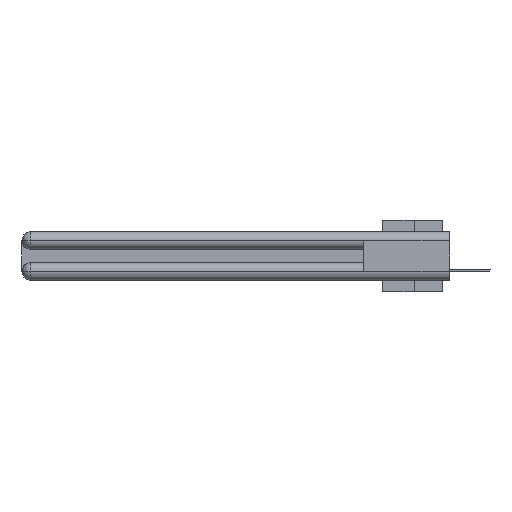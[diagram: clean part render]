
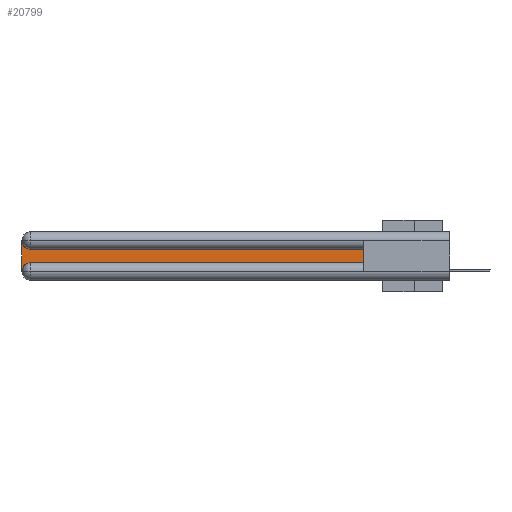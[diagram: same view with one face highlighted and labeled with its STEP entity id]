
A CAD part, left-side view. The second image highlights one B-rep face of the part: STEP entity #20799.
In plain terms, the highlighted planar face has unit normal (-1, 0, 0).
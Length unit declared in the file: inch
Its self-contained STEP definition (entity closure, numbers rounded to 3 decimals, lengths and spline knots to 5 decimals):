
#950 = VERTEX_POINT ( 'NONE', #7130 ) ;
#980 = EDGE_CURVE ( 'NONE', #950, #35146, #34189, .T. ) ;
#1785 = DIRECTION ( 'NONE',  ( 0., 0., -1. ) ) ;
#2163 = PLANE ( 'NONE',  #35764 ) ;
#2497 = CARTESIAN_POINT ( 'NONE',  ( 0.075, 2.94, -0.2175 ) ) ;
#3583 = VECTOR ( 'NONE', #12370, 39.37008 ) ;
#4427 = EDGE_CURVE ( 'NONE', #16533, #14199, #17996, .T. ) ;
#4843 = DIRECTION ( 'NONE',  ( 1., 0., 0. ) ) ;
#4846 = DIRECTION ( 'NONE',  ( 1., 0., 0. ) ) ;
#6538 = ORIENTED_EDGE ( 'NONE', *, *, #980, .T. ) ;
#7061 = LINE ( 'NONE', #24883, #12738 ) ;
#7130 = CARTESIAN_POINT ( 'NONE',  ( 0.075, 2.94, -0.1225 ) ) ;
#7988 = VERTEX_POINT ( 'NONE', #31881 ) ;
#8147 = VECTOR ( 'NONE', #15540, 39.37008 ) ;
#8931 = ORIENTED_EDGE ( 'NONE', *, *, #4427, .T. ) ;
#9205 = LINE ( 'NONE', #18027, #8147 ) ;
#10001 = EDGE_CURVE ( 'NONE', #14199, #21998, #7061, .T. ) ;
#10788 = EDGE_CURVE ( 'NONE', #21998, #7988, #30370, .T. ) ;
#12370 = DIRECTION ( 'NONE',  ( 0., 0., 1. ) ) ;
#12432 = ORIENTED_EDGE ( 'NONE', *, *, #19715, .T. ) ;
#12488 = ORIENTED_EDGE ( 'NONE', *, *, #10001, .T. ) ;
#12738 = VECTOR ( 'NONE', #19133, 39.37008 ) ;
#12980 = ORIENTED_EDGE ( 'NONE', *, *, #10788, .T. ) ;
#13119 = CARTESIAN_POINT ( 'NONE',  ( 0.075, 0.6, -0.2175 ) ) ;
#14033 = AXIS2_PLACEMENT_3D ( 'NONE', #33596, #24412, #27297 ) ;
#14199 = VERTEX_POINT ( 'NONE', #2497 ) ;
#14849 = LINE ( 'NONE', #20779, #36271 ) ;
#15540 = DIRECTION ( 'NONE',  ( 0., 1., 0. ) ) ;
#16533 = VERTEX_POINT ( 'NONE', #34102 ) ;
#17147 = DIRECTION ( 'NONE',  ( 0., 0., -1. ) ) ;
#17996 = CIRCLE ( 'NONE', #29023, 0.06 ) ;
#18027 = CARTESIAN_POINT ( 'NONE',  ( 0.075, 0.6, -0.1225 ) ) ;
#19133 = DIRECTION ( 'NONE',  ( 0., -1., 0. ) ) ;
#19715 = EDGE_CURVE ( 'NONE', #7988, #950, #9205, .T. ) ;
#20779 = CARTESIAN_POINT ( 'NONE',  ( 0.075, 3., -0.2175 ) ) ;
#20799 = ADVANCED_FACE ( 'NONE', ( #37050 ), #2163, .F. ) ;
#21998 = VERTEX_POINT ( 'NONE', #13119 ) ;
#24412 = DIRECTION ( 'NONE',  ( 1., 0., 0. ) ) ;
#24619 = CARTESIAN_POINT ( 'NONE',  ( 0.075, 2.94, -0.2775 ) ) ;
#24883 = CARTESIAN_POINT ( 'NONE',  ( 0.075, 0.6, -0.2175 ) ) ;
#27297 = DIRECTION ( 'NONE',  ( 0., 0., -1. ) ) ;
#28931 = EDGE_LOOP ( 'NONE', ( #12432, #6538, #29374, #8931, #12488, #12980 ) ) ;
#29023 = AXIS2_PLACEMENT_3D ( 'NONE', #24619, #4846, #1785 ) ;
#29374 = ORIENTED_EDGE ( 'NONE', *, *, #34319, .T. ) ;
#30011 = CARTESIAN_POINT ( 'NONE',  ( 0.075, 0.6, -0.2175 ) ) ;
#30370 = LINE ( 'NONE', #30011, #3583 ) ;
#31881 = CARTESIAN_POINT ( 'NONE',  ( 0.075, 0.6, -0.1225 ) ) ;
#32279 = DIRECTION ( 'NONE',  ( 0., 0., -1. ) ) ;
#33596 = CARTESIAN_POINT ( 'NONE',  ( 0.075, 2.94, -0.0625 ) ) ;
#34102 = CARTESIAN_POINT ( 'NONE',  ( 0.075, 3., -0.2775 ) ) ;
#34189 = CIRCLE ( 'NONE', #14033, 0.06 ) ;
#34319 = EDGE_CURVE ( 'NONE', #35146, #16533, #14849, .T. ) ;
#35146 = VERTEX_POINT ( 'NONE', #36971 ) ;
#35764 = AXIS2_PLACEMENT_3D ( 'NONE', #36667, #4843, #17147 ) ;
#36271 = VECTOR ( 'NONE', #32279, 39.37008 ) ;
#36667 = CARTESIAN_POINT ( 'NONE',  ( 0.075, 3., -0.1225 ) ) ;
#36971 = CARTESIAN_POINT ( 'NONE',  ( 0.075, 3., -0.0625 ) ) ;
#37050 = FACE_OUTER_BOUND ( 'NONE', #28931, .T. ) ;
